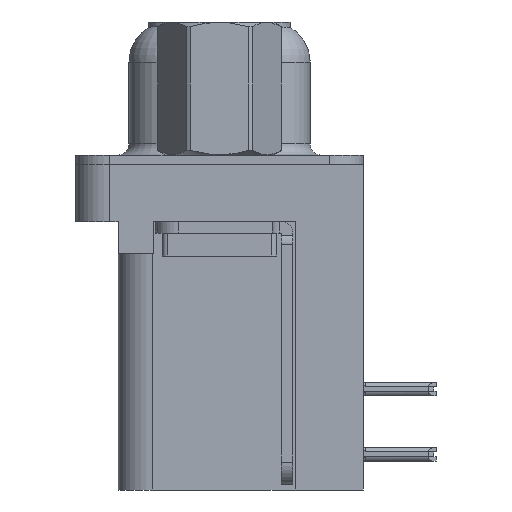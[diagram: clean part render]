
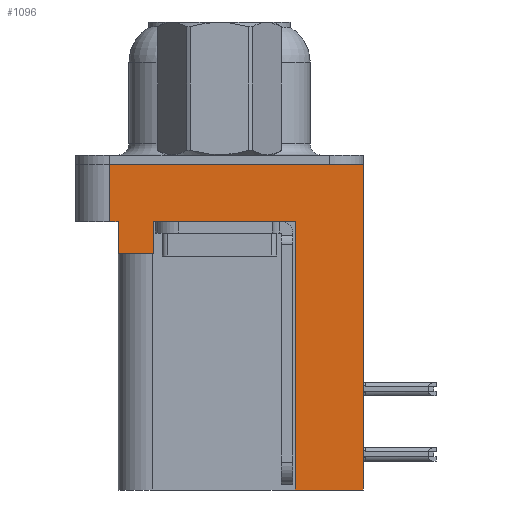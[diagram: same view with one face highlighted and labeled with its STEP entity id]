
A CAD part, left-side view. The second image highlights one B-rep face of the part: STEP entity #1096.
In plain terms, the highlighted planar face has unit normal (-1, 0, 0).
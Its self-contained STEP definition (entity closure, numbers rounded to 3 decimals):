
#170 = DIRECTION ( 'NONE',  ( 0., 0., 1. ) ) ;
#246 = ORIENTED_EDGE ( 'NONE', *, *, #28430, .F. ) ;
#534 = ORIENTED_EDGE ( 'NONE', *, *, #21723, .T. ) ;
#1096 = ADVANCED_FACE ( 'NONE', ( #9427 ), #17410, .T. ) ;
#1775 = VERTEX_POINT ( 'NONE', #2082 ) ;
#1814 = ORIENTED_EDGE ( 'NONE', *, *, #8815, .F. ) ;
#1988 = CARTESIAN_POINT ( 'NONE',  ( -3., -6.275, -2.5 ) ) ;
#2082 = CARTESIAN_POINT ( 'NONE',  ( -3., -6.275, 0. ) ) ;
#2108 = CARTESIAN_POINT ( 'NONE',  ( -3., -6.275, -2.5 ) ) ;
#2296 = VECTOR ( 'NONE', #16764, 1000. ) ;
#3607 = CARTESIAN_POINT ( 'NONE',  ( -3., 4.425, -2.5 ) ) ;
#3849 = VECTOR ( 'NONE', #170, 1000. ) ;
#4186 = VECTOR ( 'NONE', #29662, 1000. ) ;
#4360 = DIRECTION ( 'NONE',  ( -1., 0., 0. ) ) ;
#5358 = CARTESIAN_POINT ( 'NONE',  ( -3., 4.775, 0. ) ) ;
#6669 = VERTEX_POINT ( 'NONE', #9744 ) ;
#7261 = DIRECTION ( 'NONE',  ( 0., 1., 0. ) ) ;
#7416 = VECTOR ( 'NONE', #7261, 1000. ) ;
#7574 = DIRECTION ( 'NONE',  ( 0., -1., 0. ) ) ;
#8022 = ORIENTED_EDGE ( 'NONE', *, *, #33030, .F. ) ;
#8283 = VECTOR ( 'NONE', #7574, 1000. ) ;
#8660 = VERTEX_POINT ( 'NONE', #5358 ) ;
#8815 = EDGE_CURVE ( 'NONE', #23193, #19124, #11837, .T. ) ;
#8920 = DIRECTION ( 'NONE',  ( 0., -1., 0. ) ) ;
#8940 = CARTESIAN_POINT ( 'NONE',  ( -3., 4.425, -3.9 ) ) ;
#9131 = AXIS2_PLACEMENT_3D ( 'NONE', #29193, #4360, #28833 ) ;
#9339 = VERTEX_POINT ( 'NONE', #10782 ) ;
#9351 = EDGE_CURVE ( 'NONE', #6669, #9339, #16581, .T. ) ;
#9427 = FACE_OUTER_BOUND ( 'NONE', #16442, .T. ) ;
#9744 = CARTESIAN_POINT ( 'NONE',  ( -3., -3.295, -14.2 ) ) ;
#9747 = CARTESIAN_POINT ( 'NONE',  ( -3., 4.775, -2.5 ) ) ;
#10782 = CARTESIAN_POINT ( 'NONE',  ( -3., -3.295, -2.5 ) ) ;
#10858 = VECTOR ( 'NONE', #18451, 1000. ) ;
#11837 = LINE ( 'NONE', #8940, #26314 ) ;
#12701 = LINE ( 'NONE', #21214, #7416 ) ;
#12876 = CARTESIAN_POINT ( 'NONE',  ( -3., 4.775, -2.5 ) ) ;
#13559 = VECTOR ( 'NONE', #29540, 1000. ) ;
#13866 = VERTEX_POINT ( 'NONE', #34116 ) ;
#13927 = ORIENTED_EDGE ( 'NONE', *, *, #32300, .F. ) ;
#14658 = ORIENTED_EDGE ( 'NONE', *, *, #34948, .F. ) ;
#15741 = LINE ( 'NONE', #32416, #10858 ) ;
#15742 = CARTESIAN_POINT ( 'NONE',  ( -3., -6.275, -2.5 ) ) ;
#15961 = CARTESIAN_POINT ( 'NONE',  ( -3., 2.895, -3.9 ) ) ;
#16018 = CARTESIAN_POINT ( 'NONE',  ( -3., 2.895, -2.5 ) ) ;
#16442 = EDGE_LOOP ( 'NONE', ( #14658, #13927, #29074, #1814, #246, #23433, #534, #32087, #8022, #27245 ) ) ;
#16447 = EDGE_CURVE ( 'NONE', #13866, #1775, #33235, .T. ) ;
#16581 = LINE ( 'NONE', #19308, #2296 ) ;
#16764 = DIRECTION ( 'NONE',  ( 0., 0., 1. ) ) ;
#17410 = PLANE ( 'NONE',  #9131 ) ;
#18451 = DIRECTION ( 'NONE',  ( 0., 1., 0. ) ) ;
#18753 = VERTEX_POINT ( 'NONE', #12876 ) ;
#19124 = VERTEX_POINT ( 'NONE', #3607 ) ;
#19308 = CARTESIAN_POINT ( 'NONE',  ( -3., -3.295, -14.2 ) ) ;
#20607 = EDGE_CURVE ( 'NONE', #18753, #19124, #32417, .T. ) ;
#21214 = CARTESIAN_POINT ( 'NONE',  ( -3., -3.295, -14.2 ) ) ;
#21723 = EDGE_CURVE ( 'NONE', #34585, #9339, #34802, .T. ) ;
#23193 = VERTEX_POINT ( 'NONE', #27731 ) ;
#23433 = ORIENTED_EDGE ( 'NONE', *, *, #31100, .T. ) ;
#23562 = DIRECTION ( 'NONE',  ( 0., 0., 1. ) ) ;
#23672 = VECTOR ( 'NONE', #8920, 1000. ) ;
#25003 = CARTESIAN_POINT ( 'NONE',  ( -3., 2.895, -3.9 ) ) ;
#25972 = CARTESIAN_POINT ( 'NONE',  ( -3., -6.275, 0. ) ) ;
#26276 = LINE ( 'NONE', #9747, #28238 ) ;
#26314 = VECTOR ( 'NONE', #31066, 1000. ) ;
#27245 = ORIENTED_EDGE ( 'NONE', *, *, #16447, .T. ) ;
#27716 = LINE ( 'NONE', #25003, #3849 ) ;
#27731 = CARTESIAN_POINT ( 'NONE',  ( -3., 4.425, -3.9 ) ) ;
#28238 = VECTOR ( 'NONE', #23562, 1000. ) ;
#28430 = EDGE_CURVE ( 'NONE', #34094, #23193, #15741, .T. ) ;
#28833 = DIRECTION ( 'NONE',  ( 0., 0., 1. ) ) ;
#29074 = ORIENTED_EDGE ( 'NONE', *, *, #20607, .T. ) ;
#29193 = CARTESIAN_POINT ( 'NONE',  ( -3., -6.275, -2.5 ) ) ;
#29540 = DIRECTION ( 'NONE',  ( 0., -1., 0. ) ) ;
#29662 = DIRECTION ( 'NONE',  ( 0., 0., 1. ) ) ;
#31066 = DIRECTION ( 'NONE',  ( 0., 0., 1. ) ) ;
#31100 = EDGE_CURVE ( 'NONE', #34094, #34585, #27716, .T. ) ;
#32087 = ORIENTED_EDGE ( 'NONE', *, *, #9351, .F. ) ;
#32300 = EDGE_CURVE ( 'NONE', #18753, #8660, #26276, .T. ) ;
#32416 = CARTESIAN_POINT ( 'NONE',  ( -3., 4.425, -3.9 ) ) ;
#32417 = LINE ( 'NONE', #15742, #8283 ) ;
#33030 = EDGE_CURVE ( 'NONE', #13866, #6669, #12701, .T. ) ;
#33235 = LINE ( 'NONE', #2108, #4186 ) ;
#33774 = LINE ( 'NONE', #25972, #23672 ) ;
#34094 = VERTEX_POINT ( 'NONE', #15961 ) ;
#34116 = CARTESIAN_POINT ( 'NONE',  ( -3., -6.275, -14.2 ) ) ;
#34585 = VERTEX_POINT ( 'NONE', #16018 ) ;
#34802 = LINE ( 'NONE', #1988, #13559 ) ;
#34948 = EDGE_CURVE ( 'NONE', #8660, #1775, #33774, .T. ) ;
